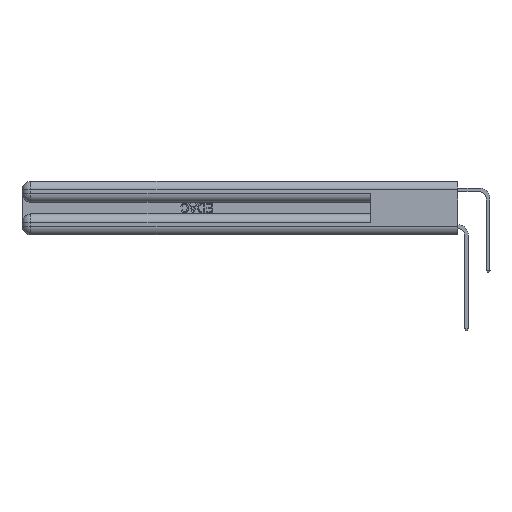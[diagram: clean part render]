
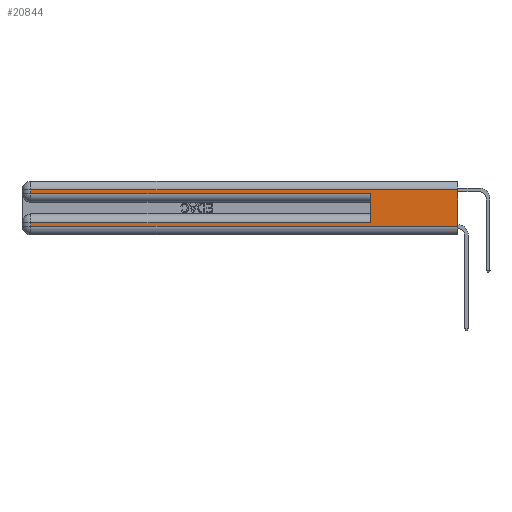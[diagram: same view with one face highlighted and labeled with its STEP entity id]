
A CAD part, left-side view. The second image highlights one B-rep face of the part: STEP entity #20844.
In plain terms, the highlighted planar face has unit normal (-1, 0, 0).
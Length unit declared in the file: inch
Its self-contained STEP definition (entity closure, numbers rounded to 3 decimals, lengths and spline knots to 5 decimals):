
#152 = VECTOR ( 'NONE', #11316, 39.37008 ) ;
#278 = DIRECTION ( 'NONE',  ( 0., 0., 1. ) ) ;
#759 = VECTOR ( 'NONE', #28919, 39.37008 ) ;
#2020 = VERTEX_POINT ( 'NONE', #10645 ) ;
#2475 = EDGE_CURVE ( 'NONE', #2020, #24203, #11877, .T. ) ;
#2571 = VERTEX_POINT ( 'NONE', #21509 ) ;
#3509 = PLANE ( 'NONE',  #3959 ) ;
#3959 = AXIS2_PLACEMENT_3D ( 'NONE', #29085, #31548, #34777 ) ;
#4458 = VECTOR ( 'NONE', #278, 39.37008 ) ;
#5411 = CARTESIAN_POINT ( 'NONE',  ( 0., 2.94, 0.37 ) ) ;
#5607 = LINE ( 'NONE', #34801, #10025 ) ;
#6123 = VECTOR ( 'NONE', #33617, 39.37008 ) ;
#6372 = ORIENTED_EDGE ( 'NONE', *, *, #13548, .F. ) ;
#8007 = LINE ( 'NONE', #19571, #6123 ) ;
#9045 = LINE ( 'NONE', #20599, #20341 ) ;
#9118 = VERTEX_POINT ( 'NONE', #14145 ) ;
#9664 = ORIENTED_EDGE ( 'NONE', *, *, #28448, .T. ) ;
#10025 = VECTOR ( 'NONE', #22877, 39.37008 ) ;
#10058 = EDGE_LOOP ( 'NONE', ( #6372, #35683, #19520, #30856, #24722, #17583, #9664, #14599 ) ) ;
#10645 = CARTESIAN_POINT ( 'NONE',  ( 0., 2.94, 0.31 ) ) ;
#10750 = CARTESIAN_POINT ( 'NONE',  ( 0., 0.6, 0.085 ) ) ;
#11316 = DIRECTION ( 'NONE',  ( 0., -1., 0. ) ) ;
#11462 = LINE ( 'NONE', #34963, #4458 ) ;
#11877 = LINE ( 'NONE', #5411, #759 ) ;
#13548 = EDGE_CURVE ( 'NONE', #2571, #28504, #21931, .T. ) ;
#14118 = EDGE_CURVE ( 'NONE', #26510, #34398, #36298, .T. ) ;
#14145 = CARTESIAN_POINT ( 'NONE',  ( 0., 0.6, 0.285 ) ) ;
#14599 = ORIENTED_EDGE ( 'NONE', *, *, #27944, .T. ) ;
#17146 = FACE_OUTER_BOUND ( 'NONE', #10058, .T. ) ;
#17583 = ORIENTED_EDGE ( 'NONE', *, *, #14118, .T. ) ;
#17824 = EDGE_CURVE ( 'NONE', #24203, #9118, #37265, .T. ) ;
#19049 = CARTESIAN_POINT ( 'NONE',  ( 0., 0., 0.085 ) ) ;
#19446 = EDGE_CURVE ( 'NONE', #26510, #9118, #11462, .T. ) ;
#19520 = ORIENTED_EDGE ( 'NONE', *, *, #2475, .T. ) ;
#19571 = CARTESIAN_POINT ( 'NONE',  ( 0., 0., 0.31 ) ) ;
#19657 = DIRECTION ( 'NONE',  ( 0., 0., -1. ) ) ;
#20341 = VECTOR ( 'NONE', #32158, 39.37008 ) ;
#20599 = CARTESIAN_POINT ( 'NONE',  ( 0., 2.94, 0.37 ) ) ;
#20844 = ADVANCED_FACE ( 'NONE', ( #17146 ), #3509, .F. ) ;
#21217 = EDGE_CURVE ( 'NONE', #2571, #2020, #8007, .T. ) ;
#21509 = CARTESIAN_POINT ( 'NONE',  ( 0., 0., 0.31 ) ) ;
#21558 = VECTOR ( 'NONE', #19657, 39.37008 ) ;
#21883 = DIRECTION ( 'NONE',  ( 0., 1., 0. ) ) ;
#21931 = LINE ( 'NONE', #33495, #21558 ) ;
#22877 = DIRECTION ( 'NONE',  ( 0., -1., 0. ) ) ;
#24203 = VERTEX_POINT ( 'NONE', #28261 ) ;
#24722 = ORIENTED_EDGE ( 'NONE', *, *, #19446, .F. ) ;
#25395 = CARTESIAN_POINT ( 'NONE',  ( 0., 2.94, 0.085 ) ) ;
#25406 = CARTESIAN_POINT ( 'NONE',  ( 0., 2.94, 0.06 ) ) ;
#26510 = VERTEX_POINT ( 'NONE', #10750 ) ;
#27944 = EDGE_CURVE ( 'NONE', #37286, #28504, #5607, .T. ) ;
#28261 = CARTESIAN_POINT ( 'NONE',  ( 0., 2.94, 0.285 ) ) ;
#28448 = EDGE_CURVE ( 'NONE', #34398, #37286, #9045, .T. ) ;
#28504 = VERTEX_POINT ( 'NONE', #30434 ) ;
#28919 = DIRECTION ( 'NONE',  ( 0., 0., -1. ) ) ;
#29085 = CARTESIAN_POINT ( 'NONE',  ( 0., 0., 0.37 ) ) ;
#30434 = CARTESIAN_POINT ( 'NONE',  ( 0., 0., 0.06 ) ) ;
#30645 = VECTOR ( 'NONE', #21883, 39.37008 ) ;
#30856 = ORIENTED_EDGE ( 'NONE', *, *, #17824, .T. ) ;
#31548 = DIRECTION ( 'NONE',  ( 1., 0., 0. ) ) ;
#32158 = DIRECTION ( 'NONE',  ( 0., 0., -1. ) ) ;
#33495 = CARTESIAN_POINT ( 'NONE',  ( 0., 0., 0.37 ) ) ;
#33617 = DIRECTION ( 'NONE',  ( 0., 1., 0. ) ) ;
#34398 = VERTEX_POINT ( 'NONE', #25395 ) ;
#34777 = DIRECTION ( 'NONE',  ( 0., 0., -1. ) ) ;
#34801 = CARTESIAN_POINT ( 'NONE',  ( 0., 0., 0.06 ) ) ;
#34963 = CARTESIAN_POINT ( 'NONE',  ( 0., 0.6, 0.145 ) ) ;
#35683 = ORIENTED_EDGE ( 'NONE', *, *, #21217, .T. ) ;
#36298 = LINE ( 'NONE', #19049, #30645 ) ;
#36886 = CARTESIAN_POINT ( 'NONE',  ( 0., 0., 0.285 ) ) ;
#37265 = LINE ( 'NONE', #36886, #152 ) ;
#37286 = VERTEX_POINT ( 'NONE', #25406 ) ;
